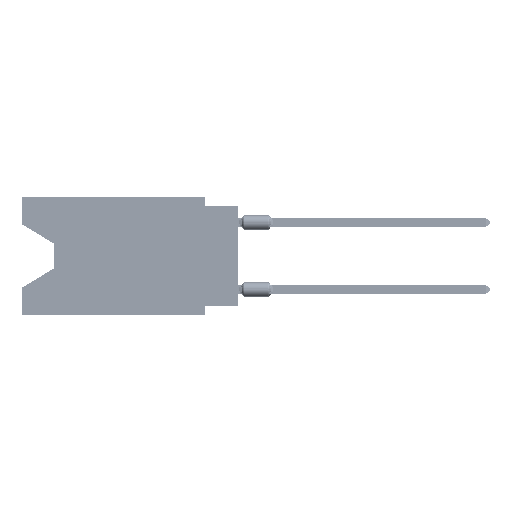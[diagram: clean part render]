
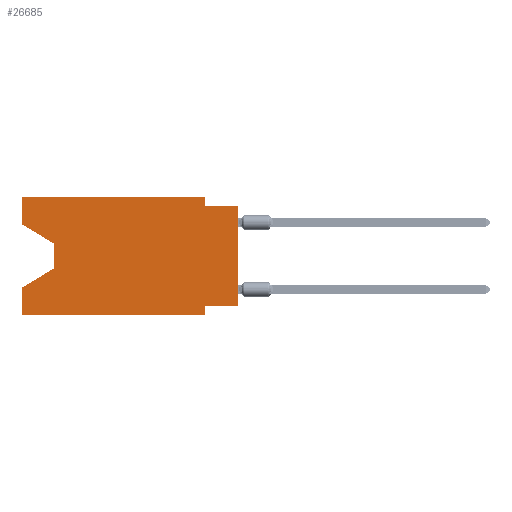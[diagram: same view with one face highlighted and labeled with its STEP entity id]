
A CAD part, left-side view. The second image highlights one B-rep face of the part: STEP entity #26685.
In plain terms, the highlighted planar face has unit normal (-1, 0, 0).
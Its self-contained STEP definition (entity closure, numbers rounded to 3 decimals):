
#24 = LINE ( 'NONE', #38605, #83975 ) ;
#469 = VERTEX_POINT ( 'NONE', #16267 ) ;
#1691 = EDGE_CURVE ( 'NONE', #31886, #52642, #98922, .T. ) ;
#2662 = VERTEX_POINT ( 'NONE', #98680 ) ;
#3206 = LINE ( 'NONE', #71751, #34609 ) ;
#6721 = AXIS2_PLACEMENT_3D ( 'NONE', #32539, #54638, #95258 ) ;
#7207 = CARTESIAN_POINT ( 'NONE',  ( 0., 2.54, 0. ) ) ;
#8791 = DIRECTION ( 'NONE',  ( 0., 0., -1. ) ) ;
#9561 = VERTEX_POINT ( 'NONE', #56575 ) ;
#11587 = VECTOR ( 'NONE', #47305, 1000. ) ;
#11954 = DIRECTION ( 'NONE',  ( 0., -1., 0. ) ) ;
#12968 = CARTESIAN_POINT ( 'NONE',  ( 0., 2.54, -8.255 ) ) ;
#13464 = LINE ( 'NONE', #21191, #71488 ) ;
#13522 = ORIENTED_EDGE ( 'NONE', *, *, #1691, .T. ) ;
#14976 = LINE ( 'NONE', #79233, #64756 ) ;
#15333 = ORIENTED_EDGE ( 'NONE', *, *, #83742, .T. ) ;
#16267 = CARTESIAN_POINT ( 'NONE',  ( 0., 2.54, -0.635 ) ) ;
#17585 = CARTESIAN_POINT ( 'NONE',  ( 0., 0., 0. ) ) ;
#18791 = EDGE_LOOP ( 'NONE', ( #13522, #68129, #20876, #21326, #15333, #84509, #33181, #28669, #57415, #73637, #72803, #60151 ) ) ;
#20037 = DIRECTION ( 'NONE',  ( 0., 0.855, -0.519 ) ) ;
#20876 = ORIENTED_EDGE ( 'NONE', *, *, #76968, .T. ) ;
#21191 = CARTESIAN_POINT ( 'NONE',  ( 0., 16.383, 0. ) ) ;
#21326 = ORIENTED_EDGE ( 'NONE', *, *, #23805, .F. ) ;
#23074 = CARTESIAN_POINT ( 'NONE',  ( 0., 0., -0.635 ) ) ;
#23805 = EDGE_CURVE ( 'NONE', #32094, #49657, #61595, .T. ) ;
#25306 = LINE ( 'NONE', #17585, #39442 ) ;
#25593 = CARTESIAN_POINT ( 'NONE',  ( 0., 16.383, 0. ) ) ;
#25879 = EDGE_CURVE ( 'NONE', #49626, #469, #92573, .T. ) ;
#26580 = DIRECTION ( 'NONE',  ( 0., 0., 1. ) ) ;
#26685 = ADVANCED_FACE ( 'NONE', ( #70582 ), #62854, .F. ) ;
#28669 = ORIENTED_EDGE ( 'NONE', *, *, #71776, .T. ) ;
#28768 = VERTEX_POINT ( 'NONE', #23074 ) ;
#30818 = EDGE_CURVE ( 'NONE', #52642, #61025, #14976, .T. ) ;
#31705 = EDGE_CURVE ( 'NONE', #78841, #66046, #65095, .T. ) ;
#31886 = VERTEX_POINT ( 'NONE', #99990 ) ;
#32094 = VERTEX_POINT ( 'NONE', #95827 ) ;
#32539 = CARTESIAN_POINT ( 'NONE',  ( 0., 16.383, 0. ) ) ;
#33181 = ORIENTED_EDGE ( 'NONE', *, *, #42881, .F. ) ;
#33232 = DIRECTION ( 'NONE',  ( 0., 0., -1. ) ) ;
#34609 = VECTOR ( 'NONE', #43805, 1000. ) ;
#35515 = EDGE_CURVE ( 'NONE', #9561, #49626, #13464, .T. ) ;
#38605 = CARTESIAN_POINT ( 'NONE',  ( 0., 0., -8.255 ) ) ;
#39194 = VECTOR ( 'NONE', #85766, 1000. ) ;
#39442 = VECTOR ( 'NONE', #48934, 1000. ) ;
#41454 = CARTESIAN_POINT ( 'NONE',  ( 0., 2.54, -8.89 ) ) ;
#41851 = VECTOR ( 'NONE', #44414, 1000. ) ;
#42881 = EDGE_CURVE ( 'NONE', #2662, #78841, #24, .T. ) ;
#43531 = VECTOR ( 'NONE', #20037, 1000. ) ;
#43805 = DIRECTION ( 'NONE',  ( 0., -1., 0. ) ) ;
#44414 = DIRECTION ( 'NONE',  ( 0., -0.855, -0.519 ) ) ;
#46265 = DIRECTION ( 'NONE',  ( 0., -1., 0. ) ) ;
#47305 = DIRECTION ( 'NONE',  ( 0., 0., -1. ) ) ;
#48934 = DIRECTION ( 'NONE',  ( 0., 0., 1. ) ) ;
#49626 = VERTEX_POINT ( 'NONE', #52428 ) ;
#49657 = VERTEX_POINT ( 'NONE', #77611 ) ;
#52428 = CARTESIAN_POINT ( 'NONE',  ( 0., 2.54, 0. ) ) ;
#52642 = VERTEX_POINT ( 'NONE', #82088 ) ;
#54638 = DIRECTION ( 'NONE',  ( 1., 0., 0. ) ) ;
#56575 = CARTESIAN_POINT ( 'NONE',  ( 0., 16.383, 0. ) ) ;
#57415 = ORIENTED_EDGE ( 'NONE', *, *, #75594, .F. ) ;
#57598 = VECTOR ( 'NONE', #26580, 1000. ) ;
#59830 = CARTESIAN_POINT ( 'NONE',  ( 0., 16.383, -2.038 ) ) ;
#60151 = ORIENTED_EDGE ( 'NONE', *, *, #92058, .F. ) ;
#61025 = VERTEX_POINT ( 'NONE', #84323 ) ;
#61091 = CARTESIAN_POINT ( 'NONE',  ( 0., 16.383, 0. ) ) ;
#61595 = LINE ( 'NONE', #61091, #39194 ) ;
#61728 = DIRECTION ( 'NONE',  ( 0., 1., 0. ) ) ;
#62854 = PLANE ( 'NONE',  #6721 ) ;
#64756 = VECTOR ( 'NONE', #8791, 1000. ) ;
#65095 = LINE ( 'NONE', #41454, #91174 ) ;
#66046 = VERTEX_POINT ( 'NONE', #89695 ) ;
#66830 = CARTESIAN_POINT ( 'NONE',  ( 0., 13.97, -5.385 ) ) ;
#68129 = ORIENTED_EDGE ( 'NONE', *, *, #30818, .T. ) ;
#70582 = FACE_OUTER_BOUND ( 'NONE', #18791, .T. ) ;
#71488 = VECTOR ( 'NONE', #11954, 1000. ) ;
#71751 = CARTESIAN_POINT ( 'NONE',  ( 0., 16.383, -8.89 ) ) ;
#71776 = EDGE_CURVE ( 'NONE', #2662, #28768, #25306, .T. ) ;
#72803 = ORIENTED_EDGE ( 'NONE', *, *, #35515, .F. ) ;
#73637 = ORIENTED_EDGE ( 'NONE', *, *, #25879, .F. ) ;
#75594 = EDGE_CURVE ( 'NONE', #469, #28768, #93558, .T. ) ;
#76968 = EDGE_CURVE ( 'NONE', #61025, #49657, #90483, .T. ) ;
#77611 = CARTESIAN_POINT ( 'NONE',  ( 0., 16.383, -6.852 ) ) ;
#77620 = CARTESIAN_POINT ( 'NONE',  ( 0., 0., -0.635 ) ) ;
#78841 = VERTEX_POINT ( 'NONE', #12968 ) ;
#79233 = CARTESIAN_POINT ( 'NONE',  ( 0., 13.97, -3.505 ) ) ;
#82088 = CARTESIAN_POINT ( 'NONE',  ( 0., 13.97, -3.505 ) ) ;
#83742 = EDGE_CURVE ( 'NONE', #32094, #66046, #3206, .T. ) ;
#83975 = VECTOR ( 'NONE', #61728, 1000. ) ;
#84323 = CARTESIAN_POINT ( 'NONE',  ( 0., 13.97, -5.385 ) ) ;
#84509 = ORIENTED_EDGE ( 'NONE', *, *, #31705, .F. ) ;
#85766 = DIRECTION ( 'NONE',  ( 0., 0., 1. ) ) ;
#89695 = CARTESIAN_POINT ( 'NONE',  ( 0., 2.54, -8.89 ) ) ;
#90483 = LINE ( 'NONE', #66830, #43531 ) ;
#91174 = VECTOR ( 'NONE', #33232, 1000. ) ;
#92058 = EDGE_CURVE ( 'NONE', #31886, #9561, #96012, .T. ) ;
#92573 = LINE ( 'NONE', #7207, #11587 ) ;
#93558 = LINE ( 'NONE', #77620, #100866 ) ;
#95258 = DIRECTION ( 'NONE',  ( 0., 0., -1. ) ) ;
#95827 = CARTESIAN_POINT ( 'NONE',  ( 0., 16.383, -8.89 ) ) ;
#96012 = LINE ( 'NONE', #25593, #57598 ) ;
#98680 = CARTESIAN_POINT ( 'NONE',  ( 0., 0., -8.255 ) ) ;
#98922 = LINE ( 'NONE', #59830, #41851 ) ;
#99990 = CARTESIAN_POINT ( 'NONE',  ( 0., 16.383, -2.038 ) ) ;
#100866 = VECTOR ( 'NONE', #46265, 1000. ) ;
